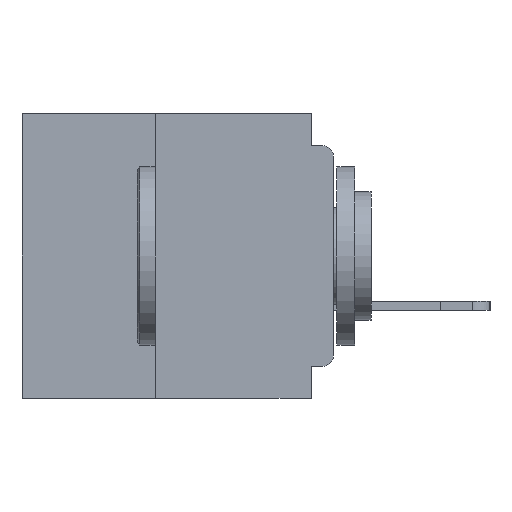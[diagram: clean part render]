
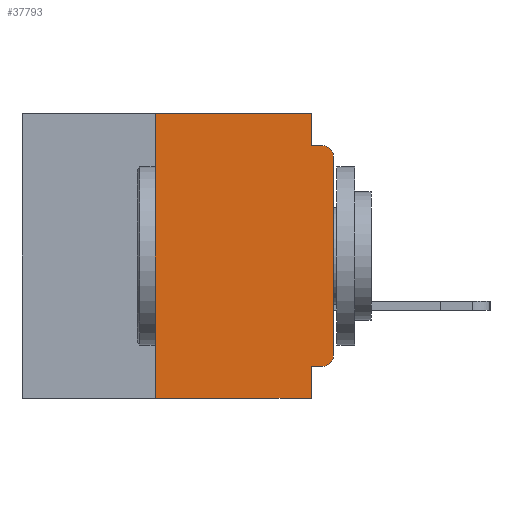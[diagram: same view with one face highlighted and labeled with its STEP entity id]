
A CAD part, left-side view. The second image highlights one B-rep face of the part: STEP entity #37793.
In plain terms, the highlighted planar face has unit normal (-1, 0, 0).
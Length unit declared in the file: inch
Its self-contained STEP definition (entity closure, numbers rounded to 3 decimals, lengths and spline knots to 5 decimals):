
#137 = EDGE_CURVE ( 'NONE', #34154, #8971, #22405, .T. ) ;
#297 = VECTOR ( 'NONE', #19155, 39.37008 ) ;
#536 = CIRCLE ( 'NONE', #7604, 0.015 ) ;
#584 = DIRECTION ( 'NONE',  ( 0., 0., -1. ) ) ;
#660 = EDGE_CURVE ( 'NONE', #13478, #15253, #536, .T. ) ;
#663 = ORIENTED_EDGE ( 'NONE', *, *, #32835, .F. ) ;
#1259 = LINE ( 'NONE', #28610, #297 ) ;
#2821 = CARTESIAN_POINT ( 'NONE',  ( 0., 0.25, 0. ) ) ;
#2867 = ORIENTED_EDGE ( 'NONE', *, *, #660, .T. ) ;
#3142 = LINE ( 'NONE', #34710, #4145 ) ;
#4145 = VECTOR ( 'NONE', #37784, 39.37008 ) ;
#4544 = VECTOR ( 'NONE', #35520, 39.37008 ) ;
#6324 = VERTEX_POINT ( 'NONE', #35479 ) ;
#6677 = CARTESIAN_POINT ( 'NONE',  ( 0., 0.031, -0.4 ) ) ;
#7043 = EDGE_CURVE ( 'NONE', #39961, #12566, #29472, .T. ) ;
#7510 = CARTESIAN_POINT ( 'NONE',  ( 0., 0.015, -0.06 ) ) ;
#7604 = AXIS2_PLACEMENT_3D ( 'NONE', #11580, #32854, #26748 ) ;
#8971 = VERTEX_POINT ( 'NONE', #11147 ) ;
#9031 = ORIENTED_EDGE ( 'NONE', *, *, #34948, .T. ) ;
#10658 = DIRECTION ( 'NONE',  ( 0., 0., -1. ) ) ;
#11147 = CARTESIAN_POINT ( 'NONE',  ( 0., 0.031, -0.045 ) ) ;
#11242 = EDGE_CURVE ( 'NONE', #13478, #6324, #15228, .T. ) ;
#11580 = CARTESIAN_POINT ( 'NONE',  ( 0., 0.015, -0.34 ) ) ;
#11626 = DIRECTION ( 'NONE',  ( 0., 1., 0. ) ) ;
#12326 = EDGE_LOOP ( 'NONE', ( #39911, #15472, #34447, #26498, #14401, #23426, #9031, #663, #36410, #2867 ) ) ;
#12566 = VERTEX_POINT ( 'NONE', #40583 ) ;
#13478 = VERTEX_POINT ( 'NONE', #22615 ) ;
#13487 = CARTESIAN_POINT ( 'NONE',  ( 0., 0.437, 0. ) ) ;
#14401 = ORIENTED_EDGE ( 'NONE', *, *, #16393, .F. ) ;
#15015 = VECTOR ( 'NONE', #584, 39.37008 ) ;
#15152 = EDGE_CURVE ( 'NONE', #15253, #39961, #1259, .T. ) ;
#15228 = LINE ( 'NONE', #33919, #16222 ) ;
#15253 = VERTEX_POINT ( 'NONE', #22770 ) ;
#15472 = ORIENTED_EDGE ( 'NONE', *, *, #7043, .T. ) ;
#16177 = VECTOR ( 'NONE', #28867, 39.37008 ) ;
#16222 = VECTOR ( 'NONE', #11626, 39.37008 ) ;
#16393 = EDGE_CURVE ( 'NONE', #29105, #34154, #3142, .T. ) ;
#17190 = LINE ( 'NONE', #19264, #16177 ) ;
#18641 = LINE ( 'NONE', #36909, #34576 ) ;
#19155 = DIRECTION ( 'NONE',  ( 0., 0., 1. ) ) ;
#19264 = CARTESIAN_POINT ( 'NONE',  ( 0., 0.25, -0.4 ) ) ;
#19902 = DIRECTION ( 'NONE',  ( 0., 0., -1. ) ) ;
#22405 = LINE ( 'NONE', #33856, #4544 ) ;
#22615 = CARTESIAN_POINT ( 'NONE',  ( 0., 0.015, -0.355 ) ) ;
#22770 = CARTESIAN_POINT ( 'NONE',  ( 0., 0., -0.34 ) ) ;
#23426 = ORIENTED_EDGE ( 'NONE', *, *, #37086, .F. ) ;
#24258 = DIRECTION ( 'NONE',  ( 0., -1., 0. ) ) ;
#24311 = CARTESIAN_POINT ( 'NONE',  ( 0., 0.25, -0.4 ) ) ;
#24890 = LINE ( 'NONE', #33893, #31349 ) ;
#26385 = CARTESIAN_POINT ( 'NONE',  ( 0., 0.031, -0.4 ) ) ;
#26498 = ORIENTED_EDGE ( 'NONE', *, *, #137, .F. ) ;
#26611 = CARTESIAN_POINT ( 'NONE',  ( 0., 0., -0.06 ) ) ;
#26748 = DIRECTION ( 'NONE',  ( 0., 0., -1. ) ) ;
#27693 = VERTEX_POINT ( 'NONE', #24311 ) ;
#28303 = EDGE_CURVE ( 'NONE', #8971, #12566, #18641, .T. ) ;
#28525 = AXIS2_PLACEMENT_3D ( 'NONE', #7510, #29714, #10658 ) ;
#28610 = CARTESIAN_POINT ( 'NONE',  ( 0., 0., 0. ) ) ;
#28867 = DIRECTION ( 'NONE',  ( 0., 0., 1. ) ) ;
#29105 = VERTEX_POINT ( 'NONE', #2821 ) ;
#29220 = PLANE ( 'NONE',  #31541 ) ;
#29472 = CIRCLE ( 'NONE', #28525, 0.015 ) ;
#29714 = DIRECTION ( 'NONE',  ( -1., 0., 0. ) ) ;
#31349 = VECTOR ( 'NONE', #37068, 39.37008 ) ;
#31541 = AXIS2_PLACEMENT_3D ( 'NONE', #13487, #38946, #19902 ) ;
#32835 = EDGE_CURVE ( 'NONE', #6324, #36590, #33002, .T. ) ;
#32845 = CARTESIAN_POINT ( 'NONE',  ( 0., 0.031, 0. ) ) ;
#32854 = DIRECTION ( 'NONE',  ( -1., 0., 0. ) ) ;
#33002 = LINE ( 'NONE', #6677, #15015 ) ;
#33420 = FACE_OUTER_BOUND ( 'NONE', #12326, .T. ) ;
#33856 = CARTESIAN_POINT ( 'NONE',  ( 0., 0.031, 0. ) ) ;
#33893 = CARTESIAN_POINT ( 'NONE',  ( 0., 0.437, -0.4 ) ) ;
#33919 = CARTESIAN_POINT ( 'NONE',  ( 0., 0., -0.355 ) ) ;
#34154 = VERTEX_POINT ( 'NONE', #32845 ) ;
#34447 = ORIENTED_EDGE ( 'NONE', *, *, #28303, .F. ) ;
#34576 = VECTOR ( 'NONE', #24258, 39.37008 ) ;
#34710 = CARTESIAN_POINT ( 'NONE',  ( 0., 0.437, 0. ) ) ;
#34948 = EDGE_CURVE ( 'NONE', #27693, #36590, #24890, .T. ) ;
#35479 = CARTESIAN_POINT ( 'NONE',  ( 0., 0.031, -0.355 ) ) ;
#35520 = DIRECTION ( 'NONE',  ( 0., 0., -1. ) ) ;
#36410 = ORIENTED_EDGE ( 'NONE', *, *, #11242, .F. ) ;
#36590 = VERTEX_POINT ( 'NONE', #26385 ) ;
#36909 = CARTESIAN_POINT ( 'NONE',  ( 0., 0., -0.045 ) ) ;
#37068 = DIRECTION ( 'NONE',  ( 0., -1., 0. ) ) ;
#37086 = EDGE_CURVE ( 'NONE', #27693, #29105, #17190, .T. ) ;
#37784 = DIRECTION ( 'NONE',  ( 0., -1., 0. ) ) ;
#37793 = ADVANCED_FACE ( 'NONE', ( #33420 ), #29220, .F. ) ;
#38946 = DIRECTION ( 'NONE',  ( 1., 0., 0. ) ) ;
#39911 = ORIENTED_EDGE ( 'NONE', *, *, #15152, .T. ) ;
#39961 = VERTEX_POINT ( 'NONE', #26611 ) ;
#40583 = CARTESIAN_POINT ( 'NONE',  ( 0., 0.015, -0.045 ) ) ;
